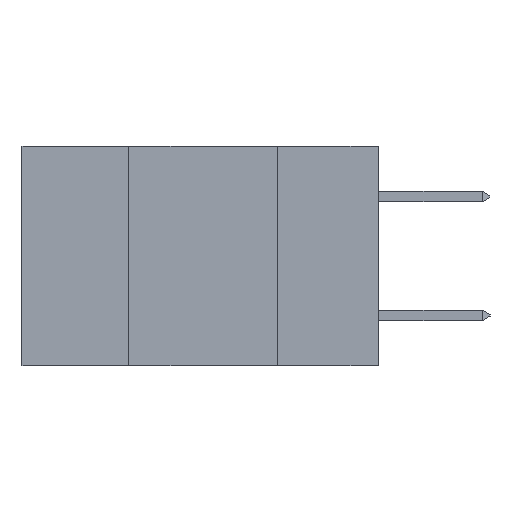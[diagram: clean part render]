
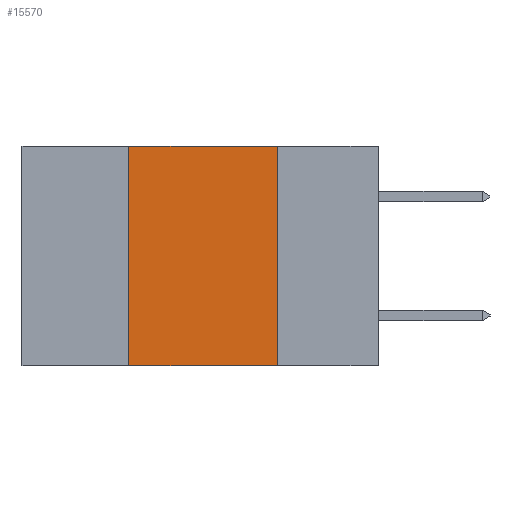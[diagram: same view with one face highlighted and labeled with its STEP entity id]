
A CAD part, left-side view. The second image highlights one B-rep face of the part: STEP entity #15570.
In plain terms, the highlighted planar face has unit normal (-1, 0, 0).
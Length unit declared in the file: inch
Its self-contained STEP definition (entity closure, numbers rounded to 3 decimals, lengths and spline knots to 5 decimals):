
#421 = DIRECTION ( 'NONE',  ( 0., 0., -1. ) ) ;
#526 = ORIENTED_EDGE ( 'NONE', *, *, #6154, .F. ) ;
#804 = EDGE_CURVE ( 'NONE', #8512, #13367, #21014, .T. ) ;
#877 = LINE ( 'NONE', #8929, #22807 ) ;
#1491 = CARTESIAN_POINT ( 'NONE',  ( 0., 0.42, 0. ) ) ;
#1647 = CARTESIAN_POINT ( 'NONE',  ( 0., 0.42, -0.37 ) ) ;
#1768 = DIRECTION ( 'NONE',  ( 0., -1., 0. ) ) ;
#1772 = VERTEX_POINT ( 'NONE', #1491 ) ;
#2809 = EDGE_CURVE ( 'NONE', #8512, #1772, #4019, .T. ) ;
#3642 = CARTESIAN_POINT ( 'NONE',  ( 0., 0.6, 0. ) ) ;
#3808 = CARTESIAN_POINT ( 'NONE',  ( 0., 0.42, -0.37 ) ) ;
#4019 = LINE ( 'NONE', #3808, #15352 ) ;
#4148 = EDGE_LOOP ( 'NONE', ( #526, #17215, #21838, #21738 ) ) ;
#5769 = PLANE ( 'NONE',  #6365 ) ;
#6154 = EDGE_CURVE ( 'NONE', #23562, #13367, #877, .T. ) ;
#6365 = AXIS2_PLACEMENT_3D ( 'NONE', #3642, #7908, #22745 ) ;
#7908 = DIRECTION ( 'NONE',  ( 1., 0., 0. ) ) ;
#8512 = VERTEX_POINT ( 'NONE', #1647 ) ;
#8929 = CARTESIAN_POINT ( 'NONE',  ( 0., 0.17, -0.37 ) ) ;
#9780 = CARTESIAN_POINT ( 'NONE',  ( 0., 0.17, -0.37 ) ) ;
#10369 = CARTESIAN_POINT ( 'NONE',  ( 0., 0.6, 0. ) ) ;
#12073 = VECTOR ( 'NONE', #1768, 39.37008 ) ;
#12214 = EDGE_CURVE ( 'NONE', #1772, #23562, #18901, .T. ) ;
#13367 = VERTEX_POINT ( 'NONE', #9780 ) ;
#14771 = FACE_OUTER_BOUND ( 'NONE', #4148, .T. ) ;
#15352 = VECTOR ( 'NONE', #20760, 39.37008 ) ;
#15570 = ADVANCED_FACE ( 'NONE', ( #14771 ), #5769, .F. ) ;
#16796 = DIRECTION ( 'NONE',  ( 0., -1., 0. ) ) ;
#17215 = ORIENTED_EDGE ( 'NONE', *, *, #12214, .F. ) ;
#18237 = CARTESIAN_POINT ( 'NONE',  ( 0., 0.6, -0.37 ) ) ;
#18248 = VECTOR ( 'NONE', #16796, 39.37008 ) ;
#18901 = LINE ( 'NONE', #10369, #18248 ) ;
#20760 = DIRECTION ( 'NONE',  ( 0., 0., 1. ) ) ;
#21014 = LINE ( 'NONE', #18237, #12073 ) ;
#21738 = ORIENTED_EDGE ( 'NONE', *, *, #804, .T. ) ;
#21838 = ORIENTED_EDGE ( 'NONE', *, *, #2809, .F. ) ;
#22290 = CARTESIAN_POINT ( 'NONE',  ( 0., 0.17, 0. ) ) ;
#22745 = DIRECTION ( 'NONE',  ( 0., 0., -1. ) ) ;
#22807 = VECTOR ( 'NONE', #421, 39.37008 ) ;
#23562 = VERTEX_POINT ( 'NONE', #22290 ) ;
